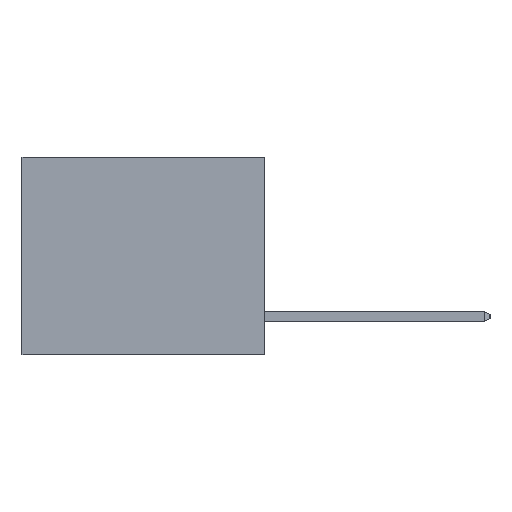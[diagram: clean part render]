
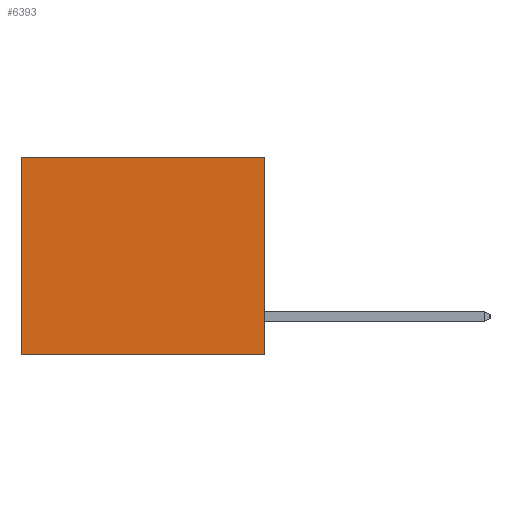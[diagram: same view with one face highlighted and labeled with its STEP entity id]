
A CAD part, left-side view. The second image highlights one B-rep face of the part: STEP entity #6393.
In plain terms, the highlighted planar face has unit normal (-1, 0, 0).
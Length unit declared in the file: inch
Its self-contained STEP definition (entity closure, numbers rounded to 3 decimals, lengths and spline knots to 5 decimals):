
#1595 = VECTOR ( 'NONE', #22222, 39.37008 ) ;
#2175 = CARTESIAN_POINT ( 'NONE',  ( 0.3165, 0., 0. ) ) ;
#2206 = ORIENTED_EDGE ( 'NONE', *, *, #7708, .F. ) ;
#2438 = CARTESIAN_POINT ( 'NONE',  ( 0.3165, 0., -0.49 ) ) ;
#4307 = LINE ( 'NONE', #17093, #24869 ) ;
#4703 = DIRECTION ( 'NONE',  ( 0., 0., -1. ) ) ;
#5469 = VERTEX_POINT ( 'NONE', #27288 ) ;
#5745 = VERTEX_POINT ( 'NONE', #6224 ) ;
#6224 = CARTESIAN_POINT ( 'NONE',  ( 0.3165, 0.6, -0.49 ) ) ;
#6393 = ADVANCED_FACE ( 'NONE', ( #7947 ), #20887, .F. ) ;
#7708 = EDGE_CURVE ( 'NONE', #19694, #13810, #22982, .T. ) ;
#7947 = FACE_OUTER_BOUND ( 'NONE', #29304, .T. ) ;
#8285 = EDGE_CURVE ( 'NONE', #19694, #5469, #15967, .T. ) ;
#9586 = CARTESIAN_POINT ( 'NONE',  ( 0.3165, 0., 0. ) ) ;
#9876 = VECTOR ( 'NONE', #10018, 39.37008 ) ;
#10018 = DIRECTION ( 'NONE',  ( 0., 1., 0. ) ) ;
#10704 = DIRECTION ( 'NONE',  ( 0., 0., -1. ) ) ;
#12422 = DIRECTION ( 'NONE',  ( 0., 1., 0. ) ) ;
#13810 = VERTEX_POINT ( 'NONE', #24729 ) ;
#14780 = AXIS2_PLACEMENT_3D ( 'NONE', #18312, #25559, #10704 ) ;
#15967 = LINE ( 'NONE', #2175, #23327 ) ;
#16460 = LINE ( 'NONE', #24648, #9876 ) ;
#17093 = CARTESIAN_POINT ( 'NONE',  ( 0.3165, 0.6, -0.49 ) ) ;
#18312 = CARTESIAN_POINT ( 'NONE',  ( 0.3165, 0., -0.49 ) ) ;
#19694 = VERTEX_POINT ( 'NONE', #9586 ) ;
#20887 = PLANE ( 'NONE',  #14780 ) ;
#21791 = ORIENTED_EDGE ( 'NONE', *, *, #8285, .T. ) ;
#22222 = DIRECTION ( 'NONE',  ( 0., 0., -1. ) ) ;
#22982 = LINE ( 'NONE', #2438, #1595 ) ;
#23327 = VECTOR ( 'NONE', #12422, 39.37008 ) ;
#24648 = CARTESIAN_POINT ( 'NONE',  ( 0.3165, 0., -0.49 ) ) ;
#24666 = ORIENTED_EDGE ( 'NONE', *, *, #26892, .T. ) ;
#24729 = CARTESIAN_POINT ( 'NONE',  ( 0.3165, 0., -0.49 ) ) ;
#24869 = VECTOR ( 'NONE', #4703, 39.37008 ) ;
#25559 = DIRECTION ( 'NONE',  ( 1., 0., 0. ) ) ;
#26892 = EDGE_CURVE ( 'NONE', #5469, #5745, #4307, .T. ) ;
#27288 = CARTESIAN_POINT ( 'NONE',  ( 0.3165, 0.6, 0. ) ) ;
#27814 = ORIENTED_EDGE ( 'NONE', *, *, #30594, .F. ) ;
#29304 = EDGE_LOOP ( 'NONE', ( #24666, #27814, #2206, #21791 ) ) ;
#30594 = EDGE_CURVE ( 'NONE', #13810, #5745, #16460, .T. ) ;
